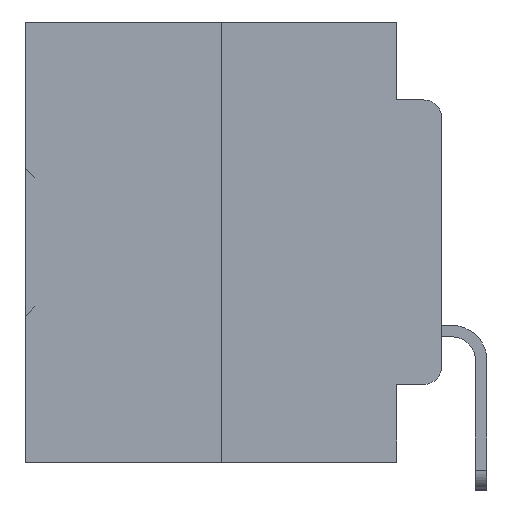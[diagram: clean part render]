
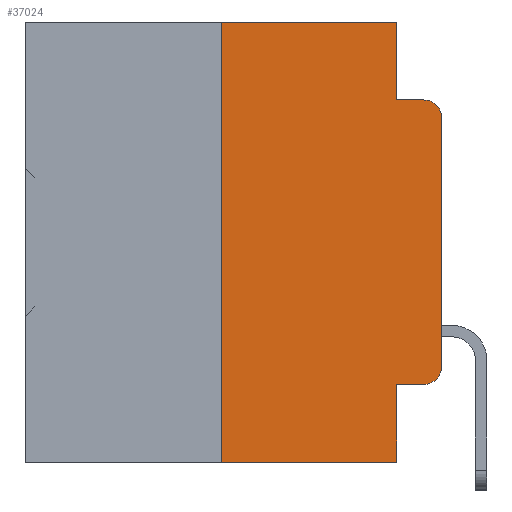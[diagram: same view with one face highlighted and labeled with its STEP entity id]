
A CAD part, left-side view. The second image highlights one B-rep face of the part: STEP entity #37024.
In plain terms, the highlighted planar face has unit normal (-1, 0, 0).
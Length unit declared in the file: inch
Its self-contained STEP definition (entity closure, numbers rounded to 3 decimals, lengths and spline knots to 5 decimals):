
#118 = DIRECTION ( 'NONE',  ( 0., 0., -1. ) ) ;
#489 = CARTESIAN_POINT ( 'NONE',  ( 0., 0.051, -0.0885 ) ) ;
#1478 = VECTOR ( 'NONE', #26058, 39.37008 ) ;
#1542 = VECTOR ( 'NONE', #31844, 39.37008 ) ;
#1764 = CIRCLE ( 'NONE', #34308, 0.02 ) ;
#2492 = LINE ( 'NONE', #13842, #1542 ) ;
#3170 = ORIENTED_EDGE ( 'NONE', *, *, #7532, .F. ) ;
#3255 = LINE ( 'NONE', #35975, #26662 ) ;
#3432 = ORIENTED_EDGE ( 'NONE', *, *, #7479, .F. ) ;
#3625 = CARTESIAN_POINT ( 'NONE',  ( 0., 0.02, -0.3915 ) ) ;
#5049 = VERTEX_POINT ( 'NONE', #13767 ) ;
#5056 = CARTESIAN_POINT ( 'NONE',  ( 0., 0.051, -0.4115 ) ) ;
#5512 = CARTESIAN_POINT ( 'NONE',  ( 0., 0., -0.3915 ) ) ;
#5740 = VERTEX_POINT ( 'NONE', #5056 ) ;
#5765 = CARTESIAN_POINT ( 'NONE',  ( 0., 0.02, -0.1085 ) ) ;
#6181 = EDGE_CURVE ( 'NONE', #23899, #38485, #28549, .T. ) ;
#6200 = CARTESIAN_POINT ( 'NONE',  ( 0., 0., 0. ) ) ;
#6729 = DIRECTION ( 'NONE',  ( 0., 0., -1. ) ) ;
#7225 = VERTEX_POINT ( 'NONE', #14115 ) ;
#7479 = EDGE_CURVE ( 'NONE', #38485, #8264, #21259, .T. ) ;
#7514 = VECTOR ( 'NONE', #30632, 39.37008 ) ;
#7532 = EDGE_CURVE ( 'NONE', #5740, #16532, #34622, .T. ) ;
#8264 = VERTEX_POINT ( 'NONE', #25077 ) ;
#8620 = VECTOR ( 'NONE', #19235, 39.37008 ) ;
#8830 = DIRECTION ( 'NONE',  ( 0., 0., -1. ) ) ;
#8893 = FACE_OUTER_BOUND ( 'NONE', #22617, .T. ) ;
#9206 = VERTEX_POINT ( 'NONE', #36346 ) ;
#9227 = PLANE ( 'NONE',  #17799 ) ;
#9733 = CARTESIAN_POINT ( 'NONE',  ( 0., 0.051, -0.5 ) ) ;
#10290 = VECTOR ( 'NONE', #12507, 39.37008 ) ;
#10732 = CARTESIAN_POINT ( 'NONE',  ( 0., 0.051, 0. ) ) ;
#12507 = DIRECTION ( 'NONE',  ( 0., 0., -1. ) ) ;
#13767 = CARTESIAN_POINT ( 'NONE',  ( 0., 0.02, -0.0885 ) ) ;
#13842 = CARTESIAN_POINT ( 'NONE',  ( 0., 0.051, -0.4115 ) ) ;
#13887 = ORIENTED_EDGE ( 'NONE', *, *, #18721, .T. ) ;
#14048 = ORIENTED_EDGE ( 'NONE', *, *, #28138, .T. ) ;
#14115 = CARTESIAN_POINT ( 'NONE',  ( 0., 0., -0.1085 ) ) ;
#14684 = LINE ( 'NONE', #6200, #7514 ) ;
#15113 = ORIENTED_EDGE ( 'NONE', *, *, #27283, .F. ) ;
#16532 = VERTEX_POINT ( 'NONE', #9733 ) ;
#16639 = CARTESIAN_POINT ( 'NONE',  ( 0., 0.25, 0. ) ) ;
#16740 = LINE ( 'NONE', #19116, #8620 ) ;
#17159 = CARTESIAN_POINT ( 'NONE',  ( 0., 0.25, -0.5 ) ) ;
#17799 = AXIS2_PLACEMENT_3D ( 'NONE', #27482, #18407, #118 ) ;
#18370 = ORIENTED_EDGE ( 'NONE', *, *, #25993, .T. ) ;
#18407 = DIRECTION ( 'NONE',  ( 1., 0., 0. ) ) ;
#18679 = LINE ( 'NONE', #10732, #1478 ) ;
#18721 = EDGE_CURVE ( 'NONE', #9206, #26815, #22615, .T. ) ;
#19116 = CARTESIAN_POINT ( 'NONE',  ( 0., 0.051, -0.0885 ) ) ;
#19235 = DIRECTION ( 'NONE',  ( 0., -1., 0. ) ) ;
#21259 = LINE ( 'NONE', #33544, #36518 ) ;
#22615 = CIRCLE ( 'NONE', #22893, 0.02 ) ;
#22617 = EDGE_LOOP ( 'NONE', ( #30282, #30884, #15113, #35014, #3432, #26248, #14048, #3170, #18370, #13887 ) ) ;
#22893 = AXIS2_PLACEMENT_3D ( 'NONE', #3625, #24981, #6729 ) ;
#23899 = VERTEX_POINT ( 'NONE', #17159 ) ;
#24981 = DIRECTION ( 'NONE',  ( -1., 0., 0. ) ) ;
#25077 = CARTESIAN_POINT ( 'NONE',  ( 0., 0.051, 0. ) ) ;
#25993 = EDGE_CURVE ( 'NONE', #5740, #9206, #2492, .T. ) ;
#26058 = DIRECTION ( 'NONE',  ( 0., 0., -1. ) ) ;
#26248 = ORIENTED_EDGE ( 'NONE', *, *, #6181, .F. ) ;
#26662 = VECTOR ( 'NONE', #39004, 39.37008 ) ;
#26815 = VERTEX_POINT ( 'NONE', #5512 ) ;
#27095 = DIRECTION ( 'NONE',  ( -1., 0., 0. ) ) ;
#27283 = EDGE_CURVE ( 'NONE', #33851, #5049, #16740, .T. ) ;
#27482 = CARTESIAN_POINT ( 'NONE',  ( 0., 0.473, 0. ) ) ;
#28138 = EDGE_CURVE ( 'NONE', #23899, #16532, #3255, .T. ) ;
#28549 = LINE ( 'NONE', #16639, #34738 ) ;
#29486 = EDGE_CURVE ( 'NONE', #7225, #5049, #1764, .T. ) ;
#30282 = ORIENTED_EDGE ( 'NONE', *, *, #36412, .T. ) ;
#30503 = DIRECTION ( 'NONE',  ( 0., -1., 0. ) ) ;
#30632 = DIRECTION ( 'NONE',  ( 0., 0., 1. ) ) ;
#30884 = ORIENTED_EDGE ( 'NONE', *, *, #29486, .T. ) ;
#31844 = DIRECTION ( 'NONE',  ( 0., -1., 0. ) ) ;
#31923 = CARTESIAN_POINT ( 'NONE',  ( 0., 0.25, 0. ) ) ;
#33544 = CARTESIAN_POINT ( 'NONE',  ( 0., 0.473, 0. ) ) ;
#33804 = CARTESIAN_POINT ( 'NONE',  ( 0., 0.051, 0. ) ) ;
#33851 = VERTEX_POINT ( 'NONE', #489 ) ;
#34308 = AXIS2_PLACEMENT_3D ( 'NONE', #5765, #27095, #8830 ) ;
#34622 = LINE ( 'NONE', #33804, #10290 ) ;
#34738 = VECTOR ( 'NONE', #37914, 39.37008 ) ;
#34746 = EDGE_CURVE ( 'NONE', #8264, #33851, #18679, .T. ) ;
#35014 = ORIENTED_EDGE ( 'NONE', *, *, #34746, .F. ) ;
#35975 = CARTESIAN_POINT ( 'NONE',  ( 0., 0.473, -0.5 ) ) ;
#36346 = CARTESIAN_POINT ( 'NONE',  ( 0., 0.02, -0.4115 ) ) ;
#36412 = EDGE_CURVE ( 'NONE', #26815, #7225, #14684, .T. ) ;
#36518 = VECTOR ( 'NONE', #30503, 39.37008 ) ;
#37024 = ADVANCED_FACE ( 'NONE', ( #8893 ), #9227, .F. ) ;
#37914 = DIRECTION ( 'NONE',  ( 0., 0., 1. ) ) ;
#38485 = VERTEX_POINT ( 'NONE', #31923 ) ;
#39004 = DIRECTION ( 'NONE',  ( 0., -1., 0. ) ) ;
